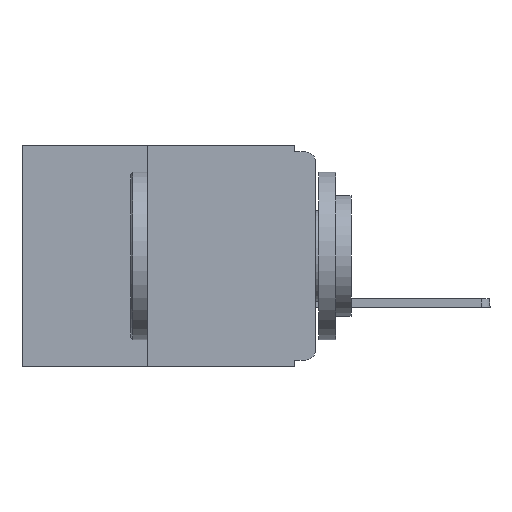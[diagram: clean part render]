
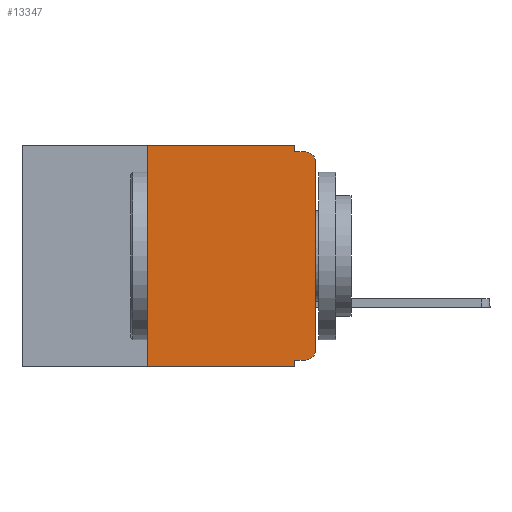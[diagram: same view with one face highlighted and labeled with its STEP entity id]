
A CAD part, left-side view. The second image highlights one B-rep face of the part: STEP entity #13347.
In plain terms, the highlighted planar face has unit normal (-1, 0, 0).
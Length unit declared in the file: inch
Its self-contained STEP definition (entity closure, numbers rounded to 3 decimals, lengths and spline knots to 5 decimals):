
#264 = CARTESIAN_POINT ( 'NONE',  ( 0., 0.015, -0.01 ) ) ;
#303 = LINE ( 'NONE', #6190, #3176 ) ;
#397 = DIRECTION ( 'NONE',  ( 0., 0., -1. ) ) ;
#1246 = DIRECTION ( 'NONE',  ( 0., 0., -1. ) ) ;
#1289 = VERTEX_POINT ( 'NONE', #13471 ) ;
#1406 = EDGE_CURVE ( 'NONE', #4554, #9547, #9044, .T. ) ;
#1455 = CARTESIAN_POINT ( 'NONE',  ( 0., 0., -0.305 ) ) ;
#1623 = CARTESIAN_POINT ( 'NONE',  ( 0., 0.031, -0.33 ) ) ;
#1649 = VECTOR ( 'NONE', #12780, 39.37008 ) ;
#1679 = ORIENTED_EDGE ( 'NONE', *, *, #8464, .T. ) ;
#1699 = ORIENTED_EDGE ( 'NONE', *, *, #9708, .T. ) ;
#1803 = ORIENTED_EDGE ( 'NONE', *, *, #12795, .F. ) ;
#1863 = CARTESIAN_POINT ( 'NONE',  ( 0., 0.25, -0.33 ) ) ;
#2057 = EDGE_CURVE ( 'NONE', #7977, #3915, #4980, .T. ) ;
#2196 = CARTESIAN_POINT ( 'NONE',  ( 0., 0.015, -0.32 ) ) ;
#2697 = VECTOR ( 'NONE', #6781, 39.37008 ) ;
#2926 = DIRECTION ( 'NONE',  ( 0., -1., 0. ) ) ;
#3031 = PLANE ( 'NONE',  #12369 ) ;
#3051 = CARTESIAN_POINT ( 'NONE',  ( 0., 0.031, 0. ) ) ;
#3090 = DIRECTION ( 'NONE',  ( 0., 0., 1. ) ) ;
#3132 = CARTESIAN_POINT ( 'NONE',  ( 0., 0., -0.025 ) ) ;
#3176 = VECTOR ( 'NONE', #12392, 39.37008 ) ;
#3212 = LINE ( 'NONE', #4335, #11900 ) ;
#3232 = EDGE_LOOP ( 'NONE', ( #1699, #5662, #7154, #12791, #11527, #1803, #1679, #4419, #10803, #6615 ) ) ;
#3672 = LINE ( 'NONE', #4826, #9677 ) ;
#3915 = VERTEX_POINT ( 'NONE', #1623 ) ;
#4335 = CARTESIAN_POINT ( 'NONE',  ( 0., 0., 0. ) ) ;
#4419 = ORIENTED_EDGE ( 'NONE', *, *, #2057, .F. ) ;
#4554 = VERTEX_POINT ( 'NONE', #2196 ) ;
#4715 = LINE ( 'NONE', #9729, #10544 ) ;
#4826 = CARTESIAN_POINT ( 'NONE',  ( 0., 0., -0.32 ) ) ;
#4980 = LINE ( 'NONE', #5977, #10456 ) ;
#5345 = CARTESIAN_POINT ( 'NONE',  ( 0., 0.015, -0.305 ) ) ;
#5427 = CARTESIAN_POINT ( 'NONE',  ( 0., 0.437, 0. ) ) ;
#5662 = ORIENTED_EDGE ( 'NONE', *, *, #11825, .T. ) ;
#5726 = DIRECTION ( 'NONE',  ( 0., 0., -1. ) ) ;
#5884 = VERTEX_POINT ( 'NONE', #10621 ) ;
#5977 = CARTESIAN_POINT ( 'NONE',  ( 0., 0.031, -0.33 ) ) ;
#6190 = CARTESIAN_POINT ( 'NONE',  ( 0., 0.437, 0. ) ) ;
#6293 = DIRECTION ( 'NONE',  ( -1., 0., 0. ) ) ;
#6318 = LINE ( 'NONE', #1863, #11600 ) ;
#6533 = DIRECTION ( 'NONE',  ( 0., 0., -1. ) ) ;
#6615 = ORIENTED_EDGE ( 'NONE', *, *, #1406, .T. ) ;
#6711 = CARTESIAN_POINT ( 'NONE',  ( 0., 0.031, 0. ) ) ;
#6742 = EDGE_CURVE ( 'NONE', #4554, #7977, #3672, .T. ) ;
#6781 = DIRECTION ( 'NONE',  ( 0., -1., 0. ) ) ;
#7154 = ORIENTED_EDGE ( 'NONE', *, *, #11952, .F. ) ;
#7942 = CARTESIAN_POINT ( 'NONE',  ( 0., 0.031, -0.32 ) ) ;
#7977 = VERTEX_POINT ( 'NONE', #7942 ) ;
#8287 = DIRECTION ( 'NONE',  ( -1., 0., 0. ) ) ;
#8325 = VERTEX_POINT ( 'NONE', #3051 ) ;
#8464 = EDGE_CURVE ( 'NONE', #5884, #3915, #13867, .T. ) ;
#8487 = AXIS2_PLACEMENT_3D ( 'NONE', #13995, #8287, #1246 ) ;
#9044 = CIRCLE ( 'NONE', #11000, 0.015 ) ;
#9425 = FACE_OUTER_BOUND ( 'NONE', #3232, .T. ) ;
#9450 = CIRCLE ( 'NONE', #8487, 0.015 ) ;
#9547 = VERTEX_POINT ( 'NONE', #1455 ) ;
#9677 = VECTOR ( 'NONE', #12211, 39.37008 ) ;
#9708 = EDGE_CURVE ( 'NONE', #9547, #11247, #3212, .T. ) ;
#9729 = CARTESIAN_POINT ( 'NONE',  ( 0., 0., -0.01 ) ) ;
#9751 = VERTEX_POINT ( 'NONE', #9990 ) ;
#9990 = CARTESIAN_POINT ( 'NONE',  ( 0., 0.031, -0.01 ) ) ;
#10166 = VERTEX_POINT ( 'NONE', #264 ) ;
#10456 = VECTOR ( 'NONE', #397, 39.37008 ) ;
#10544 = VECTOR ( 'NONE', #2926, 39.37008 ) ;
#10621 = CARTESIAN_POINT ( 'NONE',  ( 0., 0.25, -0.33 ) ) ;
#10803 = ORIENTED_EDGE ( 'NONE', *, *, #6742, .F. ) ;
#11000 = AXIS2_PLACEMENT_3D ( 'NONE', #5345, #6293, #5726 ) ;
#11247 = VERTEX_POINT ( 'NONE', #3132 ) ;
#11527 = ORIENTED_EDGE ( 'NONE', *, *, #12498, .F. ) ;
#11600 = VECTOR ( 'NONE', #3090, 39.37008 ) ;
#11825 = EDGE_CURVE ( 'NONE', #11247, #10166, #9450, .T. ) ;
#11849 = DIRECTION ( 'NONE',  ( 0., 0., 1. ) ) ;
#11900 = VECTOR ( 'NONE', #11849, 39.37008 ) ;
#11952 = EDGE_CURVE ( 'NONE', #9751, #10166, #4715, .T. ) ;
#11988 = CARTESIAN_POINT ( 'NONE',  ( 0., 0.437, -0.33 ) ) ;
#12130 = EDGE_CURVE ( 'NONE', #8325, #9751, #13142, .T. ) ;
#12211 = DIRECTION ( 'NONE',  ( 0., 1., 0. ) ) ;
#12369 = AXIS2_PLACEMENT_3D ( 'NONE', #5427, #12667, #6533 ) ;
#12392 = DIRECTION ( 'NONE',  ( 0., -1., 0. ) ) ;
#12498 = EDGE_CURVE ( 'NONE', #1289, #8325, #303, .T. ) ;
#12667 = DIRECTION ( 'NONE',  ( 1., 0., 0. ) ) ;
#12780 = DIRECTION ( 'NONE',  ( 0., 0., -1. ) ) ;
#12791 = ORIENTED_EDGE ( 'NONE', *, *, #12130, .F. ) ;
#12795 = EDGE_CURVE ( 'NONE', #5884, #1289, #6318, .T. ) ;
#13142 = LINE ( 'NONE', #6711, #1649 ) ;
#13347 = ADVANCED_FACE ( 'NONE', ( #9425 ), #3031, .F. ) ;
#13471 = CARTESIAN_POINT ( 'NONE',  ( 0., 0.25, 0. ) ) ;
#13867 = LINE ( 'NONE', #11988, #2697 ) ;
#13995 = CARTESIAN_POINT ( 'NONE',  ( 0., 0.015, -0.025 ) ) ;
